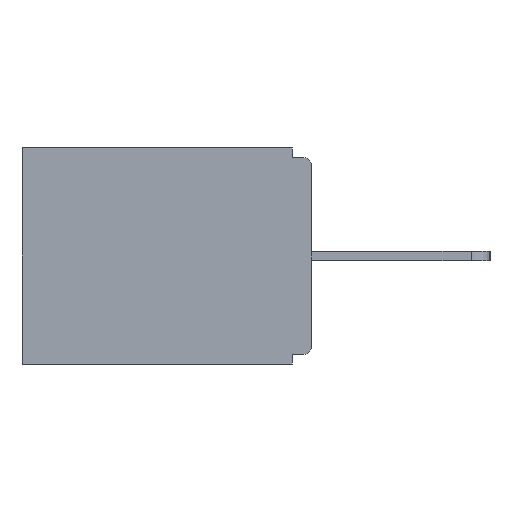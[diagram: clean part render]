
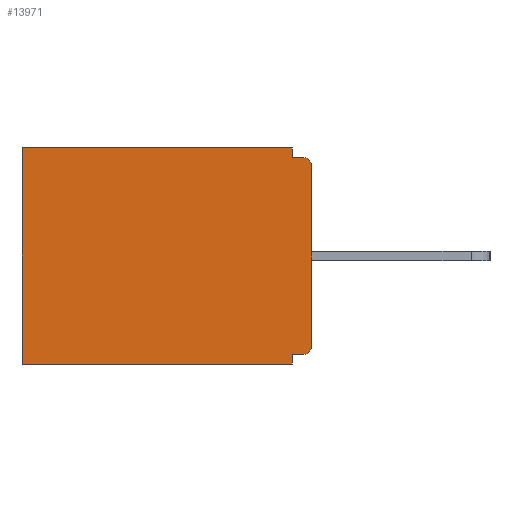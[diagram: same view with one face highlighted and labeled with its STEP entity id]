
A CAD part, left-side view. The second image highlights one B-rep face of the part: STEP entity #13971.
In plain terms, the highlighted planar face has unit normal (-1, 0, 0).
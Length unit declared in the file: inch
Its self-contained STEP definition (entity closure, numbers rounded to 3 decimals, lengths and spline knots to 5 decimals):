
#13 = AXIS2_PLACEMENT_3D ( 'NONE', #9919, #812, #11428 ) ;
#119 = CIRCLE ( 'NONE', #13, 0.015 ) ;
#750 = CIRCLE ( 'NONE', #11251, 0.015 ) ;
#812 = DIRECTION ( 'NONE',  ( -1., 0., 0. ) ) ;
#830 = DIRECTION ( 'NONE',  ( 0., -1., 0. ) ) ;
#1091 = ORIENTED_EDGE ( 'NONE', *, *, #17260, .F. ) ;
#1235 = EDGE_CURVE ( 'NONE', #8604, #1775, #15799, .T. ) ;
#1459 = VERTEX_POINT ( 'NONE', #18879 ) ;
#1663 = EDGE_CURVE ( 'NONE', #1775, #1459, #9528, .T. ) ;
#1775 = VERTEX_POINT ( 'NONE', #15136 ) ;
#1822 = VERTEX_POINT ( 'NONE', #8683 ) ;
#2968 = ORIENTED_EDGE ( 'NONE', *, *, #14125, .F. ) ;
#3229 = VERTEX_POINT ( 'NONE', #14976 ) ;
#4047 = EDGE_CURVE ( 'NONE', #8604, #6380, #12970, .T. ) ;
#4242 = DIRECTION ( 'NONE',  ( 0., 1., 0. ) ) ;
#4693 = CARTESIAN_POINT ( 'NONE',  ( 0.298, 0., -0.03 ) ) ;
#4754 = VERTEX_POINT ( 'NONE', #11918 ) ;
#5101 = VECTOR ( 'NONE', #13093, 39.37008 ) ;
#5294 = PLANE ( 'NONE',  #10360 ) ;
#5328 = FACE_OUTER_BOUND ( 'NONE', #17335, .T. ) ;
#5532 = CARTESIAN_POINT ( 'NONE',  ( 0.298, 0.031, -0.343 ) ) ;
#5630 = VERTEX_POINT ( 'NONE', #6596 ) ;
#5662 = ORIENTED_EDGE ( 'NONE', *, *, #8471, .F. ) ;
#6003 = EDGE_CURVE ( 'NONE', #16787, #5630, #18220, .T. ) ;
#6214 = DIRECTION ( 'NONE',  ( 0., 0., -1. ) ) ;
#6380 = VERTEX_POINT ( 'NONE', #8702 ) ;
#6468 = LINE ( 'NONE', #17697, #17453 ) ;
#6528 = CARTESIAN_POINT ( 'NONE',  ( 0.298, 0.46, 0. ) ) ;
#6596 = CARTESIAN_POINT ( 'NONE',  ( 0.298, 0.031, -0.328 ) ) ;
#6781 = LINE ( 'NONE', #8464, #17295 ) ;
#6829 = DIRECTION ( 'NONE',  ( 0., 0., -1. ) ) ;
#7142 = DIRECTION ( 'NONE',  ( 0., 0., -1. ) ) ;
#7291 = ORIENTED_EDGE ( 'NONE', *, *, #1235, .T. ) ;
#8044 = DIRECTION ( 'NONE',  ( 0., 1., 0. ) ) ;
#8464 = CARTESIAN_POINT ( 'NONE',  ( 0.298, 0., -0.015 ) ) ;
#8471 = EDGE_CURVE ( 'NONE', #14753, #4754, #6468, .T. ) ;
#8604 = VERTEX_POINT ( 'NONE', #13973 ) ;
#8683 = CARTESIAN_POINT ( 'NONE',  ( 0.298, 0.015, -0.015 ) ) ;
#8702 = CARTESIAN_POINT ( 'NONE',  ( 0.298, 0.031, -0.015 ) ) ;
#8720 = ORIENTED_EDGE ( 'NONE', *, *, #14686, .T. ) ;
#8795 = DIRECTION ( 'NONE',  ( -1., 0., 0. ) ) ;
#9059 = VECTOR ( 'NONE', #10350, 39.37008 ) ;
#9455 = CARTESIAN_POINT ( 'NONE',  ( 0.298, 0., 0. ) ) ;
#9519 = LINE ( 'NONE', #17203, #5101 ) ;
#9528 = LINE ( 'NONE', #6528, #9059 ) ;
#9919 = CARTESIAN_POINT ( 'NONE',  ( 0.298, 0.015, -0.03 ) ) ;
#10350 = DIRECTION ( 'NONE',  ( 0., 0., -1. ) ) ;
#10360 = AXIS2_PLACEMENT_3D ( 'NONE', #12717, #15482, #6829 ) ;
#10645 = LINE ( 'NONE', #5532, #17664 ) ;
#11251 = AXIS2_PLACEMENT_3D ( 'NONE', #17294, #8795, #18680 ) ;
#11428 = DIRECTION ( 'NONE',  ( 0., 0., -1. ) ) ;
#11766 = CARTESIAN_POINT ( 'NONE',  ( 0.298, 0.031, -0.343 ) ) ;
#11918 = CARTESIAN_POINT ( 'NONE',  ( 0.298, 0., -0.313 ) ) ;
#12113 = ORIENTED_EDGE ( 'NONE', *, *, #13434, .F. ) ;
#12717 = CARTESIAN_POINT ( 'NONE',  ( 0.298, 0., 0. ) ) ;
#12970 = LINE ( 'NONE', #11766, #16151 ) ;
#13093 = DIRECTION ( 'NONE',  ( 0., 1., 0. ) ) ;
#13415 = CARTESIAN_POINT ( 'NONE',  ( 0.298, 0., -0.328 ) ) ;
#13434 = EDGE_CURVE ( 'NONE', #6380, #1822, #6781, .T. ) ;
#13782 = ORIENTED_EDGE ( 'NONE', *, *, #1663, .T. ) ;
#13971 = ADVANCED_FACE ( 'NONE', ( #5328 ), #5294, .F. ) ;
#13973 = CARTESIAN_POINT ( 'NONE',  ( 0.298, 0.031, 0. ) ) ;
#14125 = EDGE_CURVE ( 'NONE', #3229, #1459, #9519, .T. ) ;
#14194 = VECTOR ( 'NONE', #8044, 39.37008 ) ;
#14686 = EDGE_CURVE ( 'NONE', #16787, #4754, #750, .T. ) ;
#14753 = VERTEX_POINT ( 'NONE', #4693 ) ;
#14976 = CARTESIAN_POINT ( 'NONE',  ( 0.298, 0.031, -0.343 ) ) ;
#15136 = CARTESIAN_POINT ( 'NONE',  ( 0.298, 0.46, 0. ) ) ;
#15372 = VECTOR ( 'NONE', #4242, 39.37008 ) ;
#15482 = DIRECTION ( 'NONE',  ( 1., 0., 0. ) ) ;
#15542 = DIRECTION ( 'NONE',  ( 0., 0., -1. ) ) ;
#15799 = LINE ( 'NONE', #9455, #15372 ) ;
#16151 = VECTOR ( 'NONE', #15542, 39.37008 ) ;
#16787 = VERTEX_POINT ( 'NONE', #18458 ) ;
#16853 = ORIENTED_EDGE ( 'NONE', *, *, #4047, .F. ) ;
#17203 = CARTESIAN_POINT ( 'NONE',  ( 0.298, 0., -0.343 ) ) ;
#17260 = EDGE_CURVE ( 'NONE', #5630, #3229, #10645, .T. ) ;
#17294 = CARTESIAN_POINT ( 'NONE',  ( 0.298, 0.015, -0.313 ) ) ;
#17295 = VECTOR ( 'NONE', #830, 39.37008 ) ;
#17335 = EDGE_LOOP ( 'NONE', ( #18314, #12113, #16853, #7291, #13782, #2968, #1091, #18487, #8720, #5662 ) ) ;
#17453 = VECTOR ( 'NONE', #6214, 39.37008 ) ;
#17664 = VECTOR ( 'NONE', #7142, 39.37008 ) ;
#17697 = CARTESIAN_POINT ( 'NONE',  ( 0.298, 0., 0. ) ) ;
#18220 = LINE ( 'NONE', #13415, #14194 ) ;
#18314 = ORIENTED_EDGE ( 'NONE', *, *, #18704, .T. ) ;
#18458 = CARTESIAN_POINT ( 'NONE',  ( 0.298, 0.015, -0.328 ) ) ;
#18487 = ORIENTED_EDGE ( 'NONE', *, *, #6003, .F. ) ;
#18680 = DIRECTION ( 'NONE',  ( 0., 0., -1. ) ) ;
#18704 = EDGE_CURVE ( 'NONE', #14753, #1822, #119, .T. ) ;
#18879 = CARTESIAN_POINT ( 'NONE',  ( 0.298, 0.46, -0.343 ) ) ;
